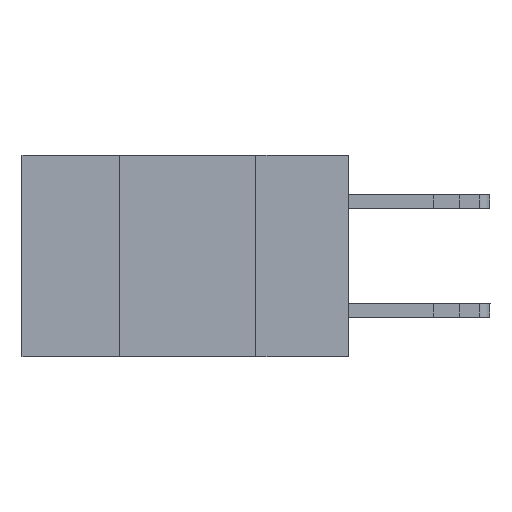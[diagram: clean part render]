
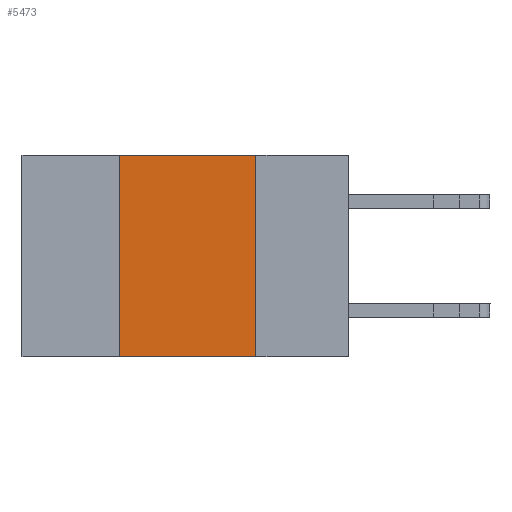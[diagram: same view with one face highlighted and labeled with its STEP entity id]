
A CAD part, left-side view. The second image highlights one B-rep face of the part: STEP entity #5473.
In plain terms, the highlighted planar face has unit normal (-1, 0, 0).
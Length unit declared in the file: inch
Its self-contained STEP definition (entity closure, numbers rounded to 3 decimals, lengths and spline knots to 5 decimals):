
#1323 = AXIS2_PLACEMENT_3D ( 'NONE', #15750, #15099, #15047 ) ;
#3763 = VECTOR ( 'NONE', #15166, 39.37008 ) ;
#4507 = VERTEX_POINT ( 'NONE', #12153 ) ;
#4581 = LINE ( 'NONE', #9160, #7582 ) ;
#5197 = LINE ( 'NONE', #8601, #8226 ) ;
#5473 = ADVANCED_FACE ( 'NONE', ( #15321 ), #15173, .F. ) ;
#5570 = EDGE_CURVE ( 'NONE', #11413, #10848, #10346, .T. ) ;
#6403 = EDGE_CURVE ( 'NONE', #10848, #4507, #14110, .T. ) ;
#6586 = VERTEX_POINT ( 'NONE', #13800 ) ;
#6861 = CARTESIAN_POINT ( 'NONE',  ( 0., 0.17, 0. ) ) ;
#7263 = EDGE_CURVE ( 'NONE', #6586, #4507, #5197, .T. ) ;
#7553 = EDGE_LOOP ( 'NONE', ( #8524, #8276, #12834, #15764 ) ) ;
#7582 = VECTOR ( 'NONE', #8750, 39.37008 ) ;
#8226 = VECTOR ( 'NONE', #8625, 39.37008 ) ;
#8276 = ORIENTED_EDGE ( 'NONE', *, *, #5570, .F. ) ;
#8524 = ORIENTED_EDGE ( 'NONE', *, *, #6403, .F. ) ;
#8601 = CARTESIAN_POINT ( 'NONE',  ( 0., 0.6, -0.37 ) ) ;
#8625 = DIRECTION ( 'NONE',  ( 0., -1., 0. ) ) ;
#8750 = DIRECTION ( 'NONE',  ( 0., 0., 1. ) ) ;
#9078 = EDGE_CURVE ( 'NONE', #6586, #11413, #4581, .T. ) ;
#9160 = CARTESIAN_POINT ( 'NONE',  ( 0., 0.42, -0.37 ) ) ;
#10346 = LINE ( 'NONE', #13914, #13323 ) ;
#10848 = VERTEX_POINT ( 'NONE', #6861 ) ;
#11413 = VERTEX_POINT ( 'NONE', #15848 ) ;
#12153 = CARTESIAN_POINT ( 'NONE',  ( 0., 0.17, -0.37 ) ) ;
#12834 = ORIENTED_EDGE ( 'NONE', *, *, #9078, .F. ) ;
#13223 = DIRECTION ( 'NONE',  ( 0., -1., 0. ) ) ;
#13323 = VECTOR ( 'NONE', #13223, 39.37008 ) ;
#13800 = CARTESIAN_POINT ( 'NONE',  ( 0., 0.42, -0.37 ) ) ;
#13914 = CARTESIAN_POINT ( 'NONE',  ( 0., 0.6, 0. ) ) ;
#14110 = LINE ( 'NONE', #15127, #3763 ) ;
#15047 = DIRECTION ( 'NONE',  ( 0., 0., -1. ) ) ;
#15099 = DIRECTION ( 'NONE',  ( 1., 0., 0. ) ) ;
#15127 = CARTESIAN_POINT ( 'NONE',  ( 0., 0.17, -0.37 ) ) ;
#15166 = DIRECTION ( 'NONE',  ( 0., 0., -1. ) ) ;
#15173 = PLANE ( 'NONE',  #1323 ) ;
#15321 = FACE_OUTER_BOUND ( 'NONE', #7553, .T. ) ;
#15750 = CARTESIAN_POINT ( 'NONE',  ( 0., 0.6, 0. ) ) ;
#15764 = ORIENTED_EDGE ( 'NONE', *, *, #7263, .T. ) ;
#15848 = CARTESIAN_POINT ( 'NONE',  ( 0., 0.42, 0. ) ) ;
